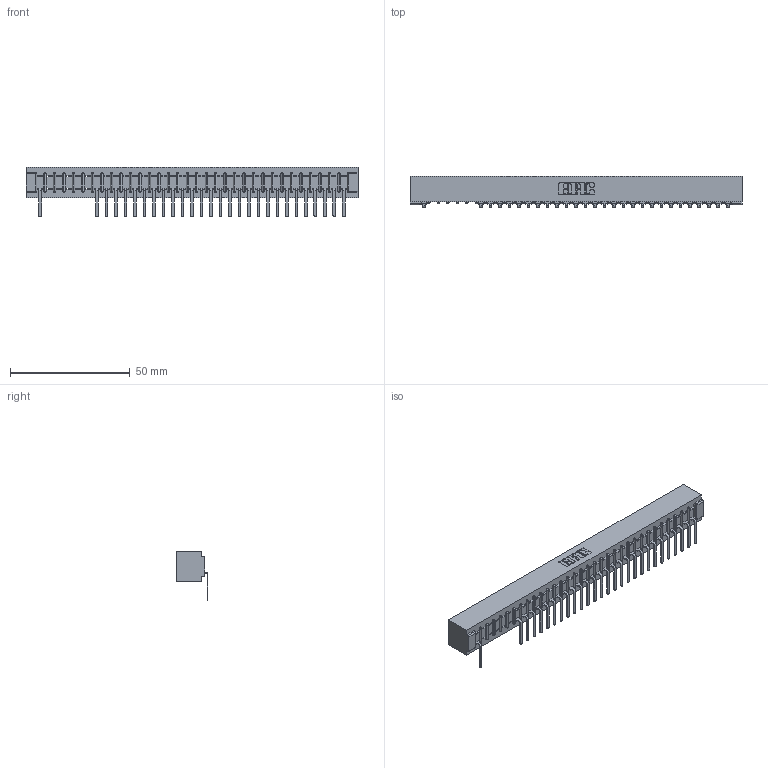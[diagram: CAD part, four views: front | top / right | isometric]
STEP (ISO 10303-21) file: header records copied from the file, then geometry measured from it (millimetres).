
FILE_DESCRIPTION (( 'STEP AP203' ), '1' );
FILE_NAME ('357-033-557-101.STEP', '2018-08-10T01:41:59', ( '' ), ( '' ), 'SwSTEP 2.0', 'SolidWorks 2016', '' );
FILE_SCHEMA (( 'CONFIG_CONTROL_DESIGN' ));
Length unit declared in the file: inch
Products named in the file (3): 307 Part_No Mounting Lugs; 307-290-002_557; 357-033-557-101
Assembly tree (29 placements, depth 2):
  357-033-557-101
    307 Part_No Mounting Lugs
    307-290-002_557  x28
Bounding box: 138.63 x 13.32 x 20.66 mm (x, y, z)
Volume: 15257 mm3; surface area: 18900.5 mm2
Topology: 29 solids, 29 shells, 2428 faces, 7451 edges, 4874 vertices
Faces by surface type: plane 1442, cylinder 918, sphere 68
Entity records: 29816 total; most frequent: CARTESIAN_POINT 5051, ORIENTED_EDGE 5046, DIRECTION 4905, EDGE_CURVE 2523, LINE 1929, VECTOR 1929, VERTEX_POINT 1634, AXIS2_PLACEMENT_3D 1488
